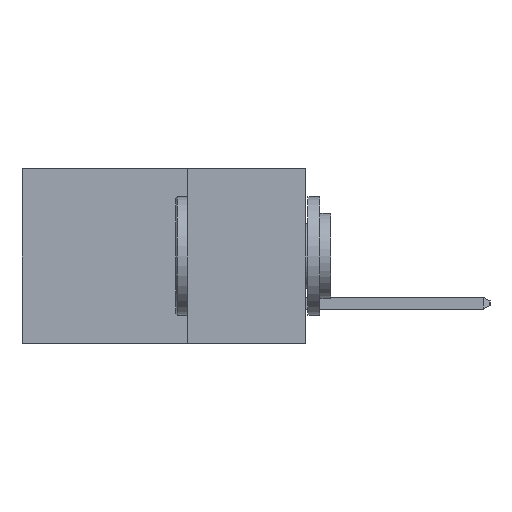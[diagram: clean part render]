
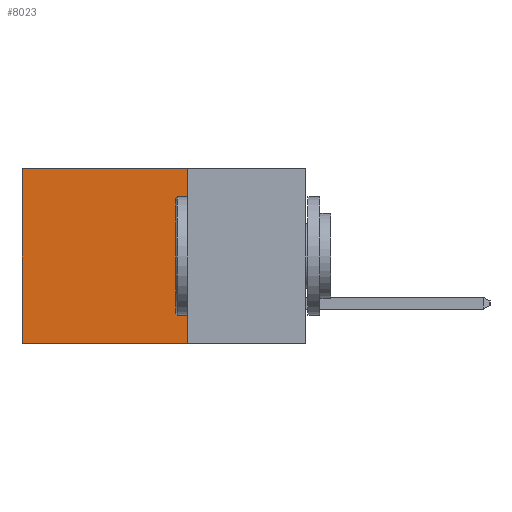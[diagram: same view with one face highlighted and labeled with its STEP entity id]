
A CAD part, left-side view. The second image highlights one B-rep face of the part: STEP entity #8023.
In plain terms, the highlighted planar face has unit normal (-1, 0, 0).
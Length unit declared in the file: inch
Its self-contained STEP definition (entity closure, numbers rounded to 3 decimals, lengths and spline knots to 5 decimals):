
#132 = DIRECTION ( 'NONE',  ( 0., 1., 0. ) ) ;
#459 = LINE ( 'NONE', #4162, #870 ) ;
#870 = VECTOR ( 'NONE', #132, 39.37008 ) ;
#966 = VERTEX_POINT ( 'NONE', #11163 ) ;
#1841 = VERTEX_POINT ( 'NONE', #9976 ) ;
#2158 = VECTOR ( 'NONE', #15828, 39.37008 ) ;
#2168 = CARTESIAN_POINT ( 'NONE',  ( 0.2615, 0.25, 0. ) ) ;
#2519 = EDGE_LOOP ( 'NONE', ( #14296, #13277, #10766, #13590 ) ) ;
#4162 = CARTESIAN_POINT ( 'NONE',  ( 0.2615, 0.25, -0.37 ) ) ;
#4758 = VECTOR ( 'NONE', #14334, 39.37008 ) ;
#4923 = PLANE ( 'NONE',  #11451 ) ;
#5532 = EDGE_CURVE ( 'NONE', #12725, #1841, #6644, .T. ) ;
#6186 = DIRECTION ( 'NONE',  ( 0., 0., -1. ) ) ;
#6369 = EDGE_CURVE ( 'NONE', #966, #6553, #459, .T. ) ;
#6553 = VERTEX_POINT ( 'NONE', #8269 ) ;
#6644 = LINE ( 'NONE', #10812, #15979 ) ;
#7334 = CARTESIAN_POINT ( 'NONE',  ( 0.2615, 0.25, -0.37 ) ) ;
#8023 = ADVANCED_FACE ( 'NONE', ( #13088 ), #4923, .F. ) ;
#8269 = CARTESIAN_POINT ( 'NONE',  ( 0.2615, 0.6, -0.37 ) ) ;
#8947 = LINE ( 'NONE', #14654, #2158 ) ;
#9976 = CARTESIAN_POINT ( 'NONE',  ( 0.2615, 0.6, 0. ) ) ;
#10376 = EDGE_CURVE ( 'NONE', #1841, #6553, #11354, .T. ) ;
#10766 = ORIENTED_EDGE ( 'NONE', *, *, #12070, .F. ) ;
#10812 = CARTESIAN_POINT ( 'NONE',  ( 0.2615, 0.25, 0. ) ) ;
#11163 = CARTESIAN_POINT ( 'NONE',  ( 0.2615, 0.25, -0.37 ) ) ;
#11354 = LINE ( 'NONE', #13119, #4758 ) ;
#11451 = AXIS2_PLACEMENT_3D ( 'NONE', #7334, #13549, #6186 ) ;
#11670 = DIRECTION ( 'NONE',  ( 0., 1., 0. ) ) ;
#12070 = EDGE_CURVE ( 'NONE', #12725, #966, #8947, .T. ) ;
#12725 = VERTEX_POINT ( 'NONE', #2168 ) ;
#13088 = FACE_OUTER_BOUND ( 'NONE', #2519, .T. ) ;
#13119 = CARTESIAN_POINT ( 'NONE',  ( 0.2615, 0.6, -0.37 ) ) ;
#13277 = ORIENTED_EDGE ( 'NONE', *, *, #6369, .F. ) ;
#13549 = DIRECTION ( 'NONE',  ( 1., 0., 0. ) ) ;
#13590 = ORIENTED_EDGE ( 'NONE', *, *, #5532, .T. ) ;
#14296 = ORIENTED_EDGE ( 'NONE', *, *, #10376, .T. ) ;
#14334 = DIRECTION ( 'NONE',  ( 0., 0., -1. ) ) ;
#14654 = CARTESIAN_POINT ( 'NONE',  ( 0.2615, 0.25, -0.37 ) ) ;
#15828 = DIRECTION ( 'NONE',  ( 0., 0., -1. ) ) ;
#15979 = VECTOR ( 'NONE', #11670, 39.37008 ) ;
